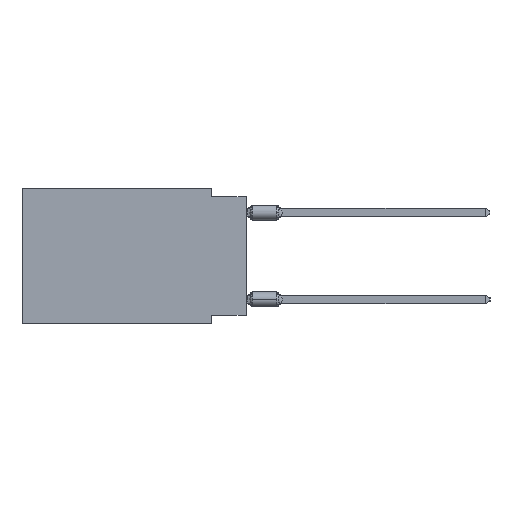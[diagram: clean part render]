
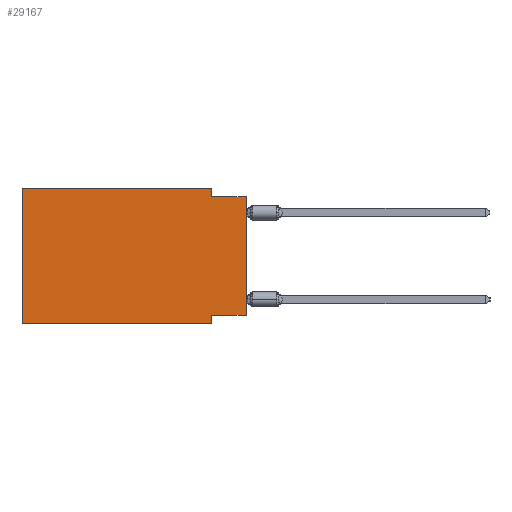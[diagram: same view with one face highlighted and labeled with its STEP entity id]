
A CAD part, left-side view. The second image highlights one B-rep face of the part: STEP entity #29167.
In plain terms, the highlighted planar face has unit normal (-1, 0, 0).
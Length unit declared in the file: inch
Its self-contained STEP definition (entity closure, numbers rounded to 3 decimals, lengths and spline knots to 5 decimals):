
#103 = EDGE_CURVE ( 'NONE', #43994, #7505, #52259, .T. ) ;
#444 = CARTESIAN_POINT ( 'NONE',  ( 0., 0.1, -0.025 ) ) ;
#1951 = LINE ( 'NONE', #41537, #56051 ) ;
#2900 = ORIENTED_EDGE ( 'NONE', *, *, #38080, .F. ) ;
#3596 = EDGE_LOOP ( 'NONE', ( #49253, #7772, #25345, #18607, #23390, #63730, #59631, #2900 ) ) ;
#5347 = VECTOR ( 'NONE', #10078, 39.37008 ) ;
#7054 = EDGE_CURVE ( 'NONE', #49420, #28933, #25188, .T. ) ;
#7505 = VERTEX_POINT ( 'NONE', #22036 ) ;
#7772 = ORIENTED_EDGE ( 'NONE', *, *, #27904, .F. ) ;
#10078 = DIRECTION ( 'NONE',  ( 0., -1., 0. ) ) ;
#10306 = CARTESIAN_POINT ( 'NONE',  ( 0., 0.645, -0.39 ) ) ;
#12047 = EDGE_CURVE ( 'NONE', #60669, #7505, #21158, .T. ) ;
#14031 = VERTEX_POINT ( 'NONE', #65096 ) ;
#16460 = CARTESIAN_POINT ( 'NONE',  ( 0., 0., -0.025 ) ) ;
#17153 = FACE_OUTER_BOUND ( 'NONE', #3596, .T. ) ;
#18353 = EDGE_CURVE ( 'NONE', #39758, #14031, #45577, .T. ) ;
#18607 = ORIENTED_EDGE ( 'NONE', *, *, #18353, .F. ) ;
#21158 = LINE ( 'NONE', #55670, #49031 ) ;
#22036 = CARTESIAN_POINT ( 'NONE',  ( 0., 0.1, -0.39 ) ) ;
#23390 = ORIENTED_EDGE ( 'NONE', *, *, #65524, .F. ) ;
#25188 = LINE ( 'NONE', #45599, #64700 ) ;
#25345 = ORIENTED_EDGE ( 'NONE', *, *, #34471, .F. ) ;
#26210 = PLANE ( 'NONE',  #30733 ) ;
#27904 = EDGE_CURVE ( 'NONE', #46301, #28933, #42229, .T. ) ;
#28933 = VERTEX_POINT ( 'NONE', #33981 ) ;
#29167 = ADVANCED_FACE ( 'NONE', ( #17153 ), #26210, .F. ) ;
#29703 = CARTESIAN_POINT ( 'NONE',  ( 0., 0.1, 0. ) ) ;
#29878 = DIRECTION ( 'NONE',  ( 0., -1., 0. ) ) ;
#29890 = CARTESIAN_POINT ( 'NONE',  ( 0., 0.1, -0.365 ) ) ;
#30733 = AXIS2_PLACEMENT_3D ( 'NONE', #62049, #37593, #46953 ) ;
#32541 = VECTOR ( 'NONE', #37734, 39.37008 ) ;
#33981 = CARTESIAN_POINT ( 'NONE',  ( 0., 0., -0.025 ) ) ;
#34471 = EDGE_CURVE ( 'NONE', #14031, #46301, #55136, .T. ) ;
#36074 = VECTOR ( 'NONE', #50123, 39.37008 ) ;
#37415 = CARTESIAN_POINT ( 'NONE',  ( 0., 0.645, 0. ) ) ;
#37593 = DIRECTION ( 'NONE',  ( 1., 0., 0. ) ) ;
#37734 = DIRECTION ( 'NONE',  ( 0., 0., 1. ) ) ;
#37828 = DIRECTION ( 'NONE',  ( 0., 1., 0. ) ) ;
#38080 = EDGE_CURVE ( 'NONE', #49420, #60669, #1951, .T. ) ;
#39758 = VERTEX_POINT ( 'NONE', #53160 ) ;
#40578 = CARTESIAN_POINT ( 'NONE',  ( 0., 0.645, 0. ) ) ;
#41537 = CARTESIAN_POINT ( 'NONE',  ( 0., 0., -0.365 ) ) ;
#41610 = CARTESIAN_POINT ( 'NONE',  ( 0., 0., -0.365 ) ) ;
#42229 = LINE ( 'NONE', #16460, #50934 ) ;
#43994 = VERTEX_POINT ( 'NONE', #10306 ) ;
#45577 = LINE ( 'NONE', #40578, #63907 ) ;
#45597 = DIRECTION ( 'NONE',  ( 0., 0., -1. ) ) ;
#45599 = CARTESIAN_POINT ( 'NONE',  ( 0., 0., 0. ) ) ;
#46267 = DIRECTION ( 'NONE',  ( 0., -1., 0. ) ) ;
#46301 = VERTEX_POINT ( 'NONE', #444 ) ;
#46953 = DIRECTION ( 'NONE',  ( 0., 0., -1. ) ) ;
#47205 = CARTESIAN_POINT ( 'NONE',  ( 0., 0.645, -0.39 ) ) ;
#49031 = VECTOR ( 'NONE', #45597, 39.37008 ) ;
#49253 = ORIENTED_EDGE ( 'NONE', *, *, #7054, .T. ) ;
#49420 = VERTEX_POINT ( 'NONE', #41610 ) ;
#50123 = DIRECTION ( 'NONE',  ( 0., 0., -1. ) ) ;
#50934 = VECTOR ( 'NONE', #46267, 39.37008 ) ;
#52259 = LINE ( 'NONE', #47205, #5347 ) ;
#53160 = CARTESIAN_POINT ( 'NONE',  ( 0., 0.645, 0. ) ) ;
#55136 = LINE ( 'NONE', #29703, #36074 ) ;
#55670 = CARTESIAN_POINT ( 'NONE',  ( 0., 0.1, -0.39 ) ) ;
#56051 = VECTOR ( 'NONE', #37828, 39.37008 ) ;
#58485 = LINE ( 'NONE', #37415, #32541 ) ;
#59631 = ORIENTED_EDGE ( 'NONE', *, *, #12047, .F. ) ;
#60669 = VERTEX_POINT ( 'NONE', #29890 ) ;
#62049 = CARTESIAN_POINT ( 'NONE',  ( 0., 0.645, 0. ) ) ;
#63730 = ORIENTED_EDGE ( 'NONE', *, *, #103, .T. ) ;
#63907 = VECTOR ( 'NONE', #29878, 39.37008 ) ;
#64700 = VECTOR ( 'NONE', #66034, 39.37008 ) ;
#65096 = CARTESIAN_POINT ( 'NONE',  ( 0., 0.1, 0. ) ) ;
#65524 = EDGE_CURVE ( 'NONE', #43994, #39758, #58485, .T. ) ;
#66034 = DIRECTION ( 'NONE',  ( 0., 0., 1. ) ) ;
